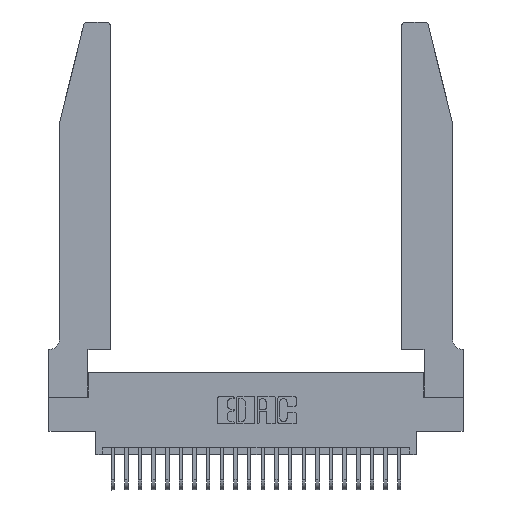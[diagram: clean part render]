
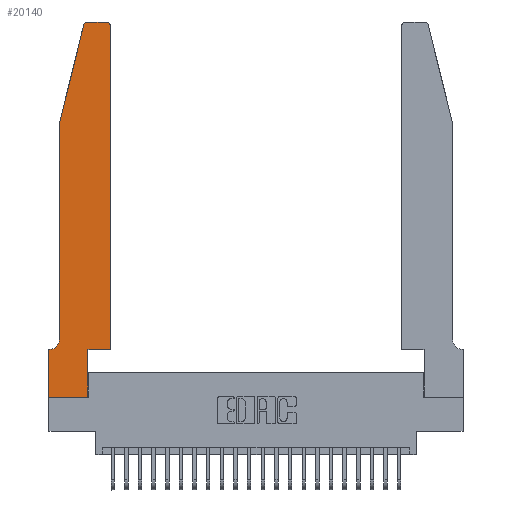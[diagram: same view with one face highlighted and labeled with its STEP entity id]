
A CAD part, top view. The second image highlights one B-rep face of the part: STEP entity #20140.
In plain terms, the highlighted planar face has unit normal (0, 0, 1).
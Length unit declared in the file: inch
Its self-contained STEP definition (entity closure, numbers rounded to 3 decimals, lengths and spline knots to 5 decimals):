
#508 = ORIENTED_EDGE ( 'NONE', *, *, #13030, .T. ) ;
#529 = LINE ( 'NONE', #6954, #9419 ) ;
#807 = DIRECTION ( 'NONE',  ( 0., 0., -1. ) ) ;
#815 = CARTESIAN_POINT ( 'NONE',  ( 0.4505, 0.35, 0.37 ) ) ;
#946 = VERTEX_POINT ( 'NONE', #19990 ) ;
#962 = PLANE ( 'NONE',  #18112 ) ;
#1917 = AXIS2_PLACEMENT_3D ( 'NONE', #12077, #807, #13938 ) ;
#2025 = VECTOR ( 'NONE', #16543, 39.37008 ) ;
#2170 = FACE_OUTER_BOUND ( 'NONE', #23784, .T. ) ;
#2265 = LINE ( 'NONE', #5628, #20921 ) ;
#2350 = CARTESIAN_POINT ( 'NONE',  ( 0., 0., 0.37 ) ) ;
#2933 = ORIENTED_EDGE ( 'NONE', *, *, #12267, .T. ) ;
#2951 = CARTESIAN_POINT ( 'NONE',  ( 0.284, 2.72, 0.37 ) ) ;
#3834 = CARTESIAN_POINT ( 'NONE',  ( 0.4205, 2.75, 0.37 ) ) ;
#4193 = VECTOR ( 'NONE', #5230, 39.37008 ) ;
#4820 = CARTESIAN_POINT ( 'NONE',  ( 0., 0.35, 0.37 ) ) ;
#4855 = DIRECTION ( 'NONE',  ( 1., 0., 0. ) ) ;
#4952 = ORIENTED_EDGE ( 'NONE', *, *, #22457, .T. ) ;
#5035 = EDGE_CURVE ( 'NONE', #12783, #946, #8635, .T. ) ;
#5156 = CARTESIAN_POINT ( 'NONE',  ( 0., 0., 0.37 ) ) ;
#5230 = DIRECTION ( 'NONE',  ( 0., 1., 0. ) ) ;
#5274 = VECTOR ( 'NONE', #21855, 39.37008 ) ;
#5451 = DIRECTION ( 'NONE',  ( -0.239, -0.971, 0. ) ) ;
#5628 = CARTESIAN_POINT ( 'NONE',  ( 0.4505, 0.35, 0.37 ) ) ;
#6160 = CARTESIAN_POINT ( 'NONE',  ( 0.4505, 2.72, 0.37 ) ) ;
#6494 = LINE ( 'NONE', #2350, #16362 ) ;
#6954 = CARTESIAN_POINT ( 'NONE',  ( 0.4505, 0.35, 0.37 ) ) ;
#7061 = LINE ( 'NONE', #23921, #2025 ) ;
#7248 = CARTESIAN_POINT ( 'NONE',  ( 0.0755, 0.42, 0.37 ) ) ;
#7561 = CARTESIAN_POINT ( 'NONE',  ( 0.2865, 0., 0.37 ) ) ;
#7794 = EDGE_CURVE ( 'NONE', #10792, #16839, #529, .T. ) ;
#7809 = VERTEX_POINT ( 'NONE', #14395 ) ;
#8010 = VERTEX_POINT ( 'NONE', #3834 ) ;
#8593 = DIRECTION ( 'NONE',  ( 1., 0., 0. ) ) ;
#8635 = CIRCLE ( 'NONE', #1917, 0.07 ) ;
#8664 = AXIS2_PLACEMENT_3D ( 'NONE', #2951, #16003, #4855 ) ;
#9419 = VECTOR ( 'NONE', #10704, 39.37008 ) ;
#9538 = VERTEX_POINT ( 'NONE', #14978 ) ;
#10085 = VERTEX_POINT ( 'NONE', #12684 ) ;
#10160 = EDGE_CURVE ( 'NONE', #10085, #13395, #16809, .T. ) ;
#10704 = DIRECTION ( 'NONE',  ( 1., 0., 0. ) ) ;
#10792 = VERTEX_POINT ( 'NONE', #12822 ) ;
#10876 = CIRCLE ( 'NONE', #8664, 0.03 ) ;
#10966 = ORIENTED_EDGE ( 'NONE', *, *, #10160, .T. ) ;
#11152 = DIRECTION ( 'NONE',  ( 0., 0., 1. ) ) ;
#11204 = VERTEX_POINT ( 'NONE', #19688 ) ;
#11879 = VECTOR ( 'NONE', #5451, 39.37008 ) ;
#12077 = CARTESIAN_POINT ( 'NONE',  ( 0.0055, 0.42, 0.37 ) ) ;
#12267 = EDGE_CURVE ( 'NONE', #22793, #10792, #18449, .T. ) ;
#12656 = CARTESIAN_POINT ( 'NONE',  ( 0.0755, 2., 0.37 ) ) ;
#12684 = CARTESIAN_POINT ( 'NONE',  ( 0.25487, 2.72718, 0.37 ) ) ;
#12783 = VERTEX_POINT ( 'NONE', #7248 ) ;
#12822 = CARTESIAN_POINT ( 'NONE',  ( 0.2865, 0.35, 0.37 ) ) ;
#12964 = CARTESIAN_POINT ( 'NONE',  ( 0.0755, 0.35, 0.37 ) ) ;
#13030 = EDGE_CURVE ( 'NONE', #7809, #22793, #6494, .T. ) ;
#13223 = AXIS2_PLACEMENT_3D ( 'NONE', #22229, #11152, #24111 ) ;
#13324 = VECTOR ( 'NONE', #22202, 39.37008 ) ;
#13395 = VERTEX_POINT ( 'NONE', #12656 ) ;
#13436 = EDGE_CURVE ( 'NONE', #13395, #12783, #21837, .T. ) ;
#13450 = EDGE_CURVE ( 'NONE', #8010, #11204, #7061, .T. ) ;
#13455 = ORIENTED_EDGE ( 'NONE', *, *, #7794, .T. ) ;
#13938 = DIRECTION ( 'NONE',  ( -1., 0., 0. ) ) ;
#14001 = EDGE_CURVE ( 'NONE', #9538, #7809, #20665, .T. ) ;
#14276 = ORIENTED_EDGE ( 'NONE', *, *, #13436, .T. ) ;
#14395 = CARTESIAN_POINT ( 'NONE',  ( 0., 0., 0.37 ) ) ;
#14978 = CARTESIAN_POINT ( 'NONE',  ( 0., 0.35, 0.37 ) ) ;
#15644 = VERTEX_POINT ( 'NONE', #6160 ) ;
#16003 = DIRECTION ( 'NONE',  ( 0., 0., 1. ) ) ;
#16333 = ORIENTED_EDGE ( 'NONE', *, *, #5035, .T. ) ;
#16362 = VECTOR ( 'NONE', #17317, 39.37008 ) ;
#16380 = CARTESIAN_POINT ( 'NONE',  ( 0.0755, 2., 0.37 ) ) ;
#16543 = DIRECTION ( 'NONE',  ( -1., 0., 0. ) ) ;
#16809 = LINE ( 'NONE', #18375, #11879 ) ;
#16839 = VERTEX_POINT ( 'NONE', #815 ) ;
#16940 = VECTOR ( 'NONE', #20195, 39.37008 ) ;
#17193 = EDGE_CURVE ( 'NONE', #15644, #8010, #23274, .T. ) ;
#17317 = DIRECTION ( 'NONE',  ( 1., 0., 0. ) ) ;
#18095 = ORIENTED_EDGE ( 'NONE', *, *, #19588, .T. ) ;
#18112 = AXIS2_PLACEMENT_3D ( 'NONE', #4820, #19691, #8593 ) ;
#18375 = CARTESIAN_POINT ( 'NONE',  ( 0.0755, 2., 0.37 ) ) ;
#18391 = EDGE_CURVE ( 'NONE', #16839, #15644, #2265, .T. ) ;
#18398 = ORIENTED_EDGE ( 'NONE', *, *, #18391, .T. ) ;
#18449 = LINE ( 'NONE', #23654, #4193 ) ;
#19551 = ORIENTED_EDGE ( 'NONE', *, *, #17193, .T. ) ;
#19588 = EDGE_CURVE ( 'NONE', #946, #9538, #23192, .T. ) ;
#19688 = CARTESIAN_POINT ( 'NONE',  ( 0.284, 2.75, 0.37 ) ) ;
#19691 = DIRECTION ( 'NONE',  ( 0., 0., 1. ) ) ;
#19824 = ORIENTED_EDGE ( 'NONE', *, *, #14001, .T. ) ;
#19990 = CARTESIAN_POINT ( 'NONE',  ( 0.0055, 0.35, 0.37 ) ) ;
#20140 = ADVANCED_FACE ( 'NONE', ( #2170 ), #962, .T. ) ;
#20195 = DIRECTION ( 'NONE',  ( 0., -1., 0. ) ) ;
#20477 = DIRECTION ( 'NONE',  ( 0., 1., 0. ) ) ;
#20665 = LINE ( 'NONE', #5156, #5274 ) ;
#20921 = VECTOR ( 'NONE', #20477, 39.37008 ) ;
#21837 = LINE ( 'NONE', #16380, #16940 ) ;
#21855 = DIRECTION ( 'NONE',  ( 0., -1., 0. ) ) ;
#22202 = DIRECTION ( 'NONE',  ( -1., 0., 0. ) ) ;
#22229 = CARTESIAN_POINT ( 'NONE',  ( 0.4205, 2.72, 0.37 ) ) ;
#22375 = ORIENTED_EDGE ( 'NONE', *, *, #13450, .T. ) ;
#22457 = EDGE_CURVE ( 'NONE', #11204, #10085, #10876, .T. ) ;
#22793 = VERTEX_POINT ( 'NONE', #7561 ) ;
#23192 = LINE ( 'NONE', #12964, #13324 ) ;
#23274 = CIRCLE ( 'NONE', #13223, 0.03 ) ;
#23654 = CARTESIAN_POINT ( 'NONE',  ( 0.2865, 0.35, 0.37 ) ) ;
#23784 = EDGE_LOOP ( 'NONE', ( #22375, #4952, #10966, #14276, #16333, #18095, #19824, #508, #2933, #13455, #18398, #19551 ) ) ;
#23921 = CARTESIAN_POINT ( 'NONE',  ( 0.2605, 2.75, 0.37 ) ) ;
#24111 = DIRECTION ( 'NONE',  ( 1., 0., 0. ) ) ;
